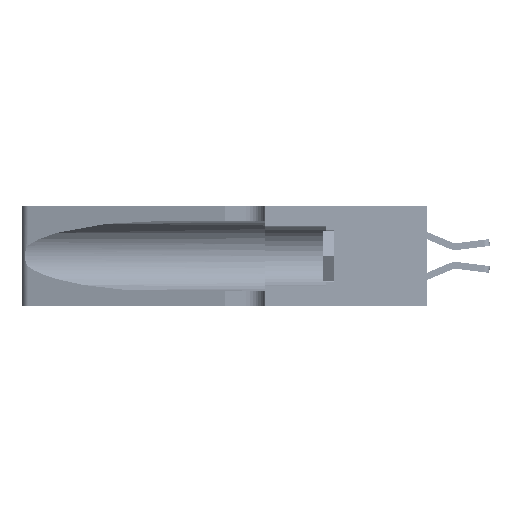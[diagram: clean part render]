
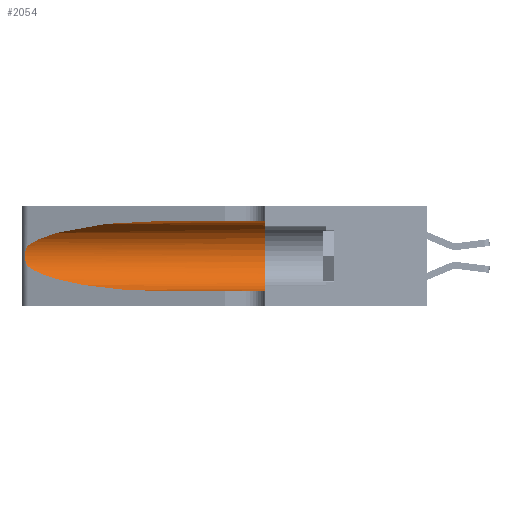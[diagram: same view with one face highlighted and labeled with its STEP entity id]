
A CAD part, left-side view. The second image highlights one B-rep face of the part: STEP entity #2054.
In plain terms, the highlighted cylindrical face has radius 3.308 mm (diameter 6.617 mm), a partial arc.
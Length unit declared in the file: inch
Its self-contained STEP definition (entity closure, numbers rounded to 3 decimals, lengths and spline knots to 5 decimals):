
#295 = CARTESIAN_POINT ( 'NONE',  ( 0.1305, 1.61858, 0.31525 ) ) ;
#447 = CARTESIAN_POINT ( 'NONE',  ( 0.25555, 1.22993, 0.14849 ) ) ;
#651 = AXIS2_PLACEMENT_3D ( 'NONE', #49162, #53099, #19326 ) ;
#1897 = CARTESIAN_POINT ( 'NONE',  ( 0.1305, 0.35, 0.31525 ) ) ;
#2054 = ADVANCED_FACE ( 'NONE', ( #22401 ), #36867, .F. ) ;
#2731 = CARTESIAN_POINT ( 'NONE',  ( 0.18966, 0.96281, 0.05475 ) ) ;
#3175 = VERTEX_POINT ( 'NONE', #49759 ) ;
#3225 = VERTEX_POINT ( 'NONE', #12470 ) ;
#4041 = DIRECTION ( 'NONE',  ( 0., 0., 1. ) ) ;
#5301 = ORIENTED_EDGE ( 'NONE', *, *, #12231, .T. ) ;
#7701 = CARTESIAN_POINT ( 'NONE',  ( 0.25487, 1.22718, 0.14631 ) ) ;
#7816 = EDGE_CURVE ( 'NONE', #45451, #3225, #50870, .T. ) ;
#8423 = CARTESIAN_POINT ( 'NONE',  ( 0.26017, 1.23833, 0.17102 ) ) ;
#10992 = VERTEX_POINT ( 'NONE', #25299 ) ;
#12231 = EDGE_CURVE ( 'NONE', #3225, #3175, #35232, .T. ) ;
#12470 = CARTESIAN_POINT ( 'NONE',  ( 0.25487, 1.22718, 0.14631 ) ) ;
#12533 = CARTESIAN_POINT ( 'NONE',  ( 0.25555, 1.22994, 0.2215 ) ) ;
#13238 = CARTESIAN_POINT ( 'NONE',  ( 0.25856, 1.23593, 0.16098 ) ) ;
#14814 = ORIENTED_EDGE ( 'NONE', *, *, #39339, .F. ) ;
#16664 = DIRECTION ( 'NONE',  ( 0., 1., 0. ) ) ;
#16960 = CARTESIAN_POINT ( 'NONE',  ( 0.25639, 1.23186, 0.15144 ) ) ;
#17519 = CARTESIAN_POINT ( 'NONE',  ( 0.25854, 1.2359, 0.20912 ) ) ;
#19326 = DIRECTION ( 'NONE',  ( 0., 0., -1. ) ) ;
#20174 = EDGE_LOOP ( 'NONE', ( #21564, #23992, #5301, #26459, #33704, #14814 ) ) ;
#21063 = CARTESIAN_POINT ( 'NONE',  ( 0.1305, 0.72297, 0.31525 ) ) ;
#21447 = CARTESIAN_POINT ( 'NONE',  ( 0.26075, 1.23896, 0.19203 ) ) ;
#21564 = ORIENTED_EDGE ( 'NONE', *, *, #45196, .T. ) ;
#21820 = CARTESIAN_POINT ( 'NONE',  ( 0.25789, 1.23486, 0.15765 ) ) ;
#21874 = EDGE_CURVE ( 'NONE', #3175, #10992, #48475, .T. ) ;
#22401 = FACE_OUTER_BOUND ( 'NONE', #20174, .T. ) ;
#23904 = AXIS2_PLACEMENT_3D ( 'NONE', #41850, #16664, #4041 ) ;
#23992 = ORIENTED_EDGE ( 'NONE', *, *, #7816, .T. ) ;
#25299 = CARTESIAN_POINT ( 'NONE',  ( 0.1305, 0.35, 0.05475 ) ) ;
#25864 = CARTESIAN_POINT ( 'NONE',  ( 0.18966, 0.96281, 0.31525 ) ) ;
#25884 = CARTESIAN_POINT ( 'NONE',  ( 0.25487, 1.22718, 0.22369 ) ) ;
#26459 = ORIENTED_EDGE ( 'NONE', *, *, #21874, .T. ) ;
#29947 = EDGE_CURVE ( 'NONE', #51347, #10992, #51612, .T. ) ;
#29992 = DIRECTION ( 'NONE',  ( 0., -1., 0. ) ) ;
#32585 = CARTESIAN_POINT ( 'NONE',  ( 0.1305, 0.72297, 0.05475 ) ) ;
#33641 = CARTESIAN_POINT ( 'NONE',  ( 0.25487, 1.22718, 0.22369 ) ) ;
#33704 = ORIENTED_EDGE ( 'NONE', *, *, #29947, .F. ) ;
#33990 = DIRECTION ( 'NONE',  ( 0., -1., 0. ) ) ;
#34027 = CARTESIAN_POINT ( 'NONE',  ( 0.25487, 1.22718, 0.14631 ) ) ;
#34349 = VERTEX_POINT ( 'NONE', #50816 ) ;
#35232 =( BOUNDED_CURVE ( )  B_SPLINE_CURVE ( 3, ( #7701, #53936, #2731, #32585 ),
 .UNSPECIFIED., .F., .T. ) 
 B_SPLINE_CURVE_WITH_KNOTS ( ( 4, 4 ),
 ( 3.44316, 4.71239 ),
 .UNSPECIFIED. ) 
 CURVE ( )  GEOMETRIC_REPRESENTATION_ITEM ( )  RATIONAL_B_SPLINE_CURVE ( ( 1., 0.87, 0.87, 1. ) ) 
 REPRESENTATION_ITEM ( '' )  );
#36867 = CYLINDRICAL_SURFACE ( 'NONE', #651, 0.13025 ) ;
#37195 = VECTOR ( 'NONE', #33990, 39.37008 ) ;
#38607 = CARTESIAN_POINT ( 'NONE',  ( 0.1305, 1.61858, 0.05475 ) ) ;
#39339 = EDGE_CURVE ( 'NONE', #34349, #51347, #44575, .T. ) ;
#41850 = CARTESIAN_POINT ( 'NONE',  ( 0.1305, 0.35, 0.185 ) ) ;
#41927 = VECTOR ( 'NONE', #29992, 39.37008 ) ;
#42152 = CARTESIAN_POINT ( 'NONE',  ( 0.25639, 1.23184, 0.21858 ) ) ;
#42718 = CARTESIAN_POINT ( 'NONE',  ( 0.26075, 1.23896, 0.178 ) ) ;
#44575 = LINE ( 'NONE', #295, #41927 ) ;
#45196 = EDGE_CURVE ( 'NONE', #34349, #45451, #52612, .T. ) ;
#45451 = VERTEX_POINT ( 'NONE', #47521 ) ;
#46424 = CARTESIAN_POINT ( 'NONE',  ( 0.26018, 1.23835, 0.19895 ) ) ;
#46782 = CARTESIAN_POINT ( 'NONE',  ( 0.25787, 1.23484, 0.2124 ) ) ;
#47521 = CARTESIAN_POINT ( 'NONE',  ( 0.25487, 1.22718, 0.22369 ) ) ;
#48475 = LINE ( 'NONE', #38607, #37195 ) ;
#49162 = CARTESIAN_POINT ( 'NONE',  ( 0.1305, 1.61858, 0.185 ) ) ;
#49759 = CARTESIAN_POINT ( 'NONE',  ( 0.1305, 0.72297, 0.05475 ) ) ;
#50707 = CARTESIAN_POINT ( 'NONE',  ( 0.2373, 1.15595, 0.28018 ) ) ;
#50816 = CARTESIAN_POINT ( 'NONE',  ( 0.1305, 0.72297, 0.31525 ) ) ;
#50870 = B_SPLINE_CURVE_WITH_KNOTS ( 'NONE', 3,
 ( #25884, #12533, #42152, #46782, #17519, #46424, #21447, #42718, #8423, #13238, #21820, #16960, #447, #34027 ),
 .UNSPECIFIED., .F., .F.,
 ( 4, 2, 2, 2, 2, 2, 4 ),
 ( 0., 0.00027, 0.00053, 0.00107, 0.0016, 0.00187, 0.00214 ),
 .UNSPECIFIED. ) ;
#51347 = VERTEX_POINT ( 'NONE', #1897 ) ;
#51612 = CIRCLE ( 'NONE', #23904, 0.13025 ) ;
#52612 =( BOUNDED_CURVE ( )  B_SPLINE_CURVE ( 3, ( #21063, #25864, #50707, #33641 ),
 .UNSPECIFIED., .F., .F. ) 
 B_SPLINE_CURVE_WITH_KNOTS ( ( 4, 4 ),
 ( 1.5708, 2.84003 ),
 .UNSPECIFIED. ) 
 CURVE ( )  GEOMETRIC_REPRESENTATION_ITEM ( )  RATIONAL_B_SPLINE_CURVE ( ( 1., 0.87, 0.87, 1. ) ) 
 REPRESENTATION_ITEM ( '' )  );
#53099 = DIRECTION ( 'NONE',  ( 0., -1., 0. ) ) ;
#53936 = CARTESIAN_POINT ( 'NONE',  ( 0.2373, 1.15595, 0.08982 ) ) ;
